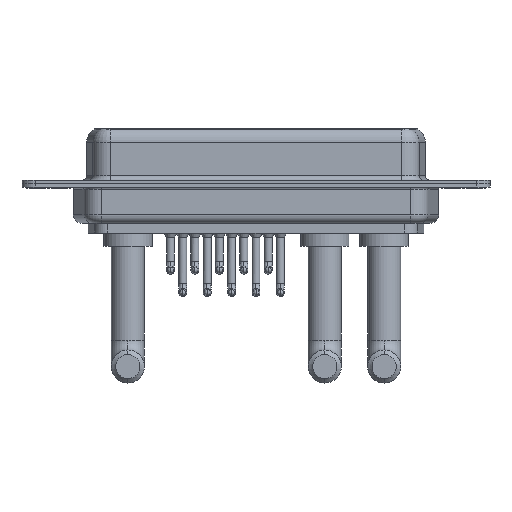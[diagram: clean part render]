
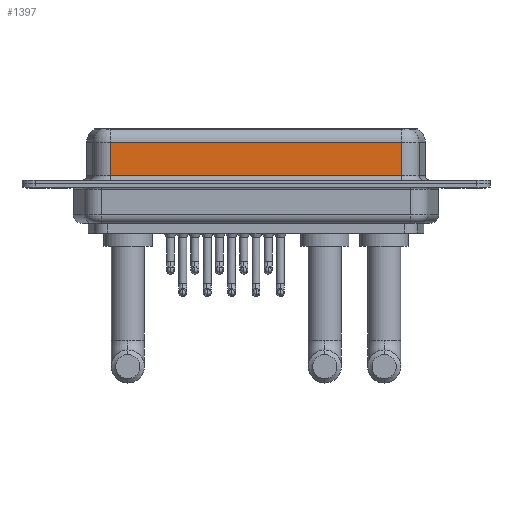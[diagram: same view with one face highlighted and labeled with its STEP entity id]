
A CAD part, front view. The second image highlights one B-rep face of the part: STEP entity #1397.
In plain terms, the highlighted planar face has unit normal (0, -1, 0).
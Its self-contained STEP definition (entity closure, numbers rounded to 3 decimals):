
#357 = VECTOR ( 'NONE', #5364, 1000. ) ;
#1174 = CARTESIAN_POINT ( 'NONE',  ( 40.037, -3.95, 0.9 ) ) ;
#1309 = PLANE ( 'NONE',  #1344 ) ;
#1344 = AXIS2_PLACEMENT_3D ( 'NONE', #10891, #8015, #13267 ) ;
#1397 = ADVANCED_FACE ( 'NONE', ( #5565 ), #1309, .F. ) ;
#1446 = CARTESIAN_POINT ( 'NONE',  ( 7.013, -3.95, 6.4 ) ) ;
#2420 = VERTEX_POINT ( 'NONE', #12937 ) ;
#2590 = CARTESIAN_POINT ( 'NONE',  ( 40.037, -3.95, 6.4 ) ) ;
#2743 = DIRECTION ( 'NONE',  ( 1., 0., 0. ) ) ;
#3045 = VERTEX_POINT ( 'NONE', #14639 ) ;
#3416 = EDGE_CURVE ( 'NONE', #9822, #14120, #10509, .T. ) ;
#5364 = DIRECTION ( 'NONE',  ( 0., 0., -1. ) ) ;
#5565 = FACE_OUTER_BOUND ( 'NONE', #16579, .T. ) ;
#5883 = VECTOR ( 'NONE', #12105, 1000. ) ;
#6038 = EDGE_CURVE ( 'NONE', #3045, #2420, #10768, .T. ) ;
#6345 = CARTESIAN_POINT ( 'NONE',  ( 40.037, -3.95, 0.9 ) ) ;
#6859 = LINE ( 'NONE', #2590, #5883 ) ;
#7184 = VECTOR ( 'NONE', #11895, 1000. ) ;
#8015 = DIRECTION ( 'NONE',  ( 0., 1., 0. ) ) ;
#8051 = CARTESIAN_POINT ( 'NONE',  ( 40.037, -3.95, 4.65 ) ) ;
#8339 = ORIENTED_EDGE ( 'NONE', *, *, #10159, .T. ) ;
#9012 = ORIENTED_EDGE ( 'NONE', *, *, #3416, .T. ) ;
#9337 = VECTOR ( 'NONE', #2743, 1000. ) ;
#9435 = ORIENTED_EDGE ( 'NONE', *, *, #6038, .T. ) ;
#9822 = VERTEX_POINT ( 'NONE', #10540 ) ;
#10159 = EDGE_CURVE ( 'NONE', #2420, #9822, #12090, .T. ) ;
#10509 = LINE ( 'NONE', #1174, #9337 ) ;
#10540 = CARTESIAN_POINT ( 'NONE',  ( 7.013, -3.95, 0.9 ) ) ;
#10768 = LINE ( 'NONE', #8051, #7184 ) ;
#10891 = CARTESIAN_POINT ( 'NONE',  ( 40.037, -3.95, 6.4 ) ) ;
#11895 = DIRECTION ( 'NONE',  ( -1., 0., 0. ) ) ;
#12090 = LINE ( 'NONE', #1446, #357 ) ;
#12105 = DIRECTION ( 'NONE',  ( 0., 0., -1. ) ) ;
#12937 = CARTESIAN_POINT ( 'NONE',  ( 7.013, -3.95, 4.65 ) ) ;
#12970 = EDGE_CURVE ( 'NONE', #3045, #14120, #6859, .T. ) ;
#13267 = DIRECTION ( 'NONE',  ( 0., 0., 1. ) ) ;
#14120 = VERTEX_POINT ( 'NONE', #6345 ) ;
#14639 = CARTESIAN_POINT ( 'NONE',  ( 40.037, -3.95, 4.65 ) ) ;
#16579 = EDGE_LOOP ( 'NONE', ( #16679, #9435, #8339, #9012 ) ) ;
#16679 = ORIENTED_EDGE ( 'NONE', *, *, #12970, .F. ) ;
